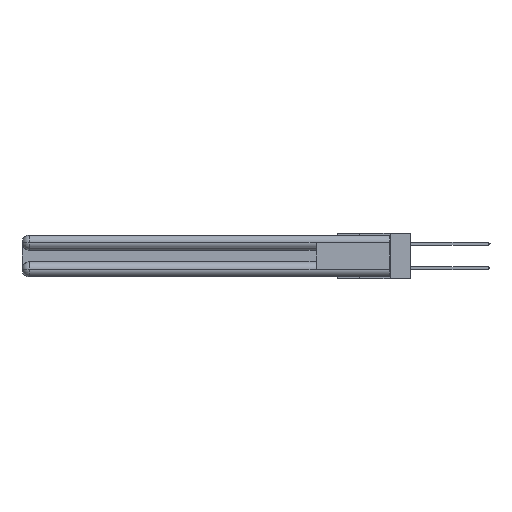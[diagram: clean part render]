
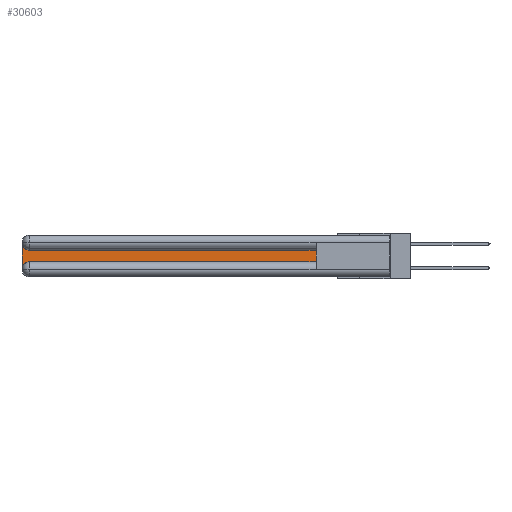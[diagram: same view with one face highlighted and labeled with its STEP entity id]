
A CAD part, left-side view. The second image highlights one B-rep face of the part: STEP entity #30603.
In plain terms, the highlighted planar face has unit normal (-1, 0, 0).
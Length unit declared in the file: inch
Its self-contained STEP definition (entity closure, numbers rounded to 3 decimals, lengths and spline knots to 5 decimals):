
#827 = ORIENTED_EDGE ( 'NONE', *, *, #18886, .T. ) ;
#1151 = CARTESIAN_POINT ( 'NONE',  ( 0.075, 3., -0.2775 ) ) ;
#1488 = VERTEX_POINT ( 'NONE', #29101 ) ;
#1619 = VERTEX_POINT ( 'NONE', #1151 ) ;
#2119 = DIRECTION ( 'NONE',  ( 0., 1., 0. ) ) ;
#2345 = PLANE ( 'NONE',  #12032 ) ;
#4139 = VERTEX_POINT ( 'NONE', #6789 ) ;
#4774 = ORIENTED_EDGE ( 'NONE', *, *, #12879, .T. ) ;
#5375 = VERTEX_POINT ( 'NONE', #19475 ) ;
#6153 = DIRECTION ( 'NONE',  ( 0., 0., -1. ) ) ;
#6251 = ORIENTED_EDGE ( 'NONE', *, *, #27744, .T. ) ;
#6789 = CARTESIAN_POINT ( 'NONE',  ( 0.075, 0.6, -0.1225 ) ) ;
#9334 = FACE_OUTER_BOUND ( 'NONE', #26952, .T. ) ;
#9852 = DIRECTION ( 'NONE',  ( 1., 0., 0. ) ) ;
#10750 = DIRECTION ( 'NONE',  ( 0., 0., -1. ) ) ;
#11010 = DIRECTION ( 'NONE',  ( 1., 0., 0. ) ) ;
#11535 = DIRECTION ( 'NONE',  ( 0., -1., 0. ) ) ;
#12032 = AXIS2_PLACEMENT_3D ( 'NONE', #25008, #9852, #19931 ) ;
#12398 = VERTEX_POINT ( 'NONE', #17150 ) ;
#12879 = EDGE_CURVE ( 'NONE', #12398, #5375, #31806, .T. ) ;
#14176 = CARTESIAN_POINT ( 'NONE',  ( 0.075, 0.6, -0.2175 ) ) ;
#14476 = VECTOR ( 'NONE', #26756, 39.37008 ) ;
#15504 = CARTESIAN_POINT ( 'NONE',  ( 0.075, 2.94, -0.0625 ) ) ;
#16324 = CARTESIAN_POINT ( 'NONE',  ( 0.075, 2.94, -0.2775 ) ) ;
#16343 = CARTESIAN_POINT ( 'NONE',  ( 0.075, 3., -0.2175 ) ) ;
#17150 = CARTESIAN_POINT ( 'NONE',  ( 0.075, 2.94, -0.2175 ) ) ;
#18533 = AXIS2_PLACEMENT_3D ( 'NONE', #15504, #31005, #10750 ) ;
#18886 = EDGE_CURVE ( 'NONE', #1619, #12398, #27024, .T. ) ;
#18961 = VERTEX_POINT ( 'NONE', #31052 ) ;
#19475 = CARTESIAN_POINT ( 'NONE',  ( 0.075, 0.6, -0.2175 ) ) ;
#19931 = DIRECTION ( 'NONE',  ( 0., 0., -1. ) ) ;
#20171 = LINE ( 'NONE', #27400, #22971 ) ;
#20776 = EDGE_CURVE ( 'NONE', #5375, #4139, #20171, .T. ) ;
#21951 = VECTOR ( 'NONE', #2119, 39.37008 ) ;
#22540 = CIRCLE ( 'NONE', #18533, 0.06 ) ;
#22971 = VECTOR ( 'NONE', #32380, 39.37008 ) ;
#23879 = VECTOR ( 'NONE', #11535, 39.37008 ) ;
#24973 = AXIS2_PLACEMENT_3D ( 'NONE', #16324, #11010, #6153 ) ;
#25008 = CARTESIAN_POINT ( 'NONE',  ( 0.075, 3., -0.1225 ) ) ;
#25059 = EDGE_CURVE ( 'NONE', #1488, #18961, #22540, .T. ) ;
#26756 = DIRECTION ( 'NONE',  ( 0., 0., -1. ) ) ;
#26952 = EDGE_LOOP ( 'NONE', ( #30952, #28626, #6251, #827, #4774, #30010 ) ) ;
#27024 = CIRCLE ( 'NONE', #24973, 0.06 ) ;
#27400 = CARTESIAN_POINT ( 'NONE',  ( 0.075, 0.6, -0.2175 ) ) ;
#27744 = EDGE_CURVE ( 'NONE', #18961, #1619, #27944, .T. ) ;
#27885 = LINE ( 'NONE', #29825, #21951 ) ;
#27944 = LINE ( 'NONE', #16343, #14476 ) ;
#28626 = ORIENTED_EDGE ( 'NONE', *, *, #25059, .T. ) ;
#29101 = CARTESIAN_POINT ( 'NONE',  ( 0.075, 2.94, -0.1225 ) ) ;
#29825 = CARTESIAN_POINT ( 'NONE',  ( 0.075, 0.6, -0.1225 ) ) ;
#30010 = ORIENTED_EDGE ( 'NONE', *, *, #20776, .T. ) ;
#30603 = ADVANCED_FACE ( 'NONE', ( #9334 ), #2345, .F. ) ;
#30952 = ORIENTED_EDGE ( 'NONE', *, *, #31957, .T. ) ;
#31005 = DIRECTION ( 'NONE',  ( 1., 0., 0. ) ) ;
#31052 = CARTESIAN_POINT ( 'NONE',  ( 0.075, 3., -0.0625 ) ) ;
#31806 = LINE ( 'NONE', #14176, #23879 ) ;
#31957 = EDGE_CURVE ( 'NONE', #4139, #1488, #27885, .T. ) ;
#32380 = DIRECTION ( 'NONE',  ( 0., 0., 1. ) ) ;
